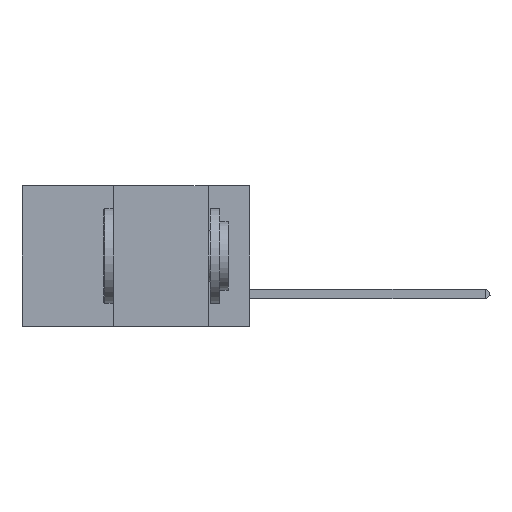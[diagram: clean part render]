
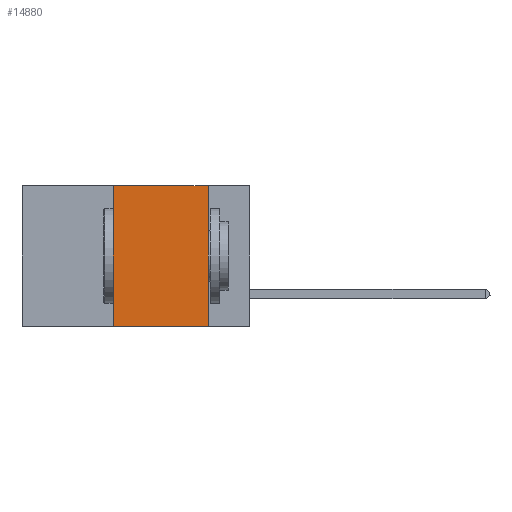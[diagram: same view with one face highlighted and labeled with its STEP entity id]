
A CAD part, left-side view. The second image highlights one B-rep face of the part: STEP entity #14880.
In plain terms, the highlighted planar face has unit normal (-1, 0, 0).
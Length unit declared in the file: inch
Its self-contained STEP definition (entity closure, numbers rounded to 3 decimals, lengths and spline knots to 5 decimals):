
#73 = CARTESIAN_POINT ( 'NONE',  ( 0., 0.11, 0. ) ) ;
#715 = CARTESIAN_POINT ( 'NONE',  ( 0., 0.36, 0. ) ) ;
#4609 = VERTEX_POINT ( 'NONE', #715 ) ;
#6145 = CARTESIAN_POINT ( 'NONE',  ( 0., 0.11, 0. ) ) ;
#11748 = EDGE_CURVE ( 'NONE', #20192, #26360, #21008, .T. ) ;
#11791 = CARTESIAN_POINT ( 'NONE',  ( 0., 0.6, 0. ) ) ;
#12547 = VECTOR ( 'NONE', #41056, 39.37008 ) ;
#13272 = DIRECTION ( 'NONE',  ( 0., -1., 0. ) ) ;
#14880 = ADVANCED_FACE ( 'NONE', ( #40308 ), #36085, .F. ) ;
#18778 = CARTESIAN_POINT ( 'NONE',  ( 0., 0.36, -0.37 ) ) ;
#19255 = CARTESIAN_POINT ( 'NONE',  ( 0., 0.11, -0.37 ) ) ;
#20192 = VERTEX_POINT ( 'NONE', #18778 ) ;
#21008 = LINE ( 'NONE', #24125, #21643 ) ;
#21636 = EDGE_CURVE ( 'NONE', #31765, #26360, #34710, .T. ) ;
#21643 = VECTOR ( 'NONE', #13272, 39.37008 ) ;
#22984 = EDGE_LOOP ( 'NONE', ( #28183, #44640, #44623, #33241 ) ) ;
#24125 = CARTESIAN_POINT ( 'NONE',  ( 0., 0.6, -0.37 ) ) ;
#24415 = AXIS2_PLACEMENT_3D ( 'NONE', #28059, #35913, #43634 ) ;
#26360 = VERTEX_POINT ( 'NONE', #19255 ) ;
#28059 = CARTESIAN_POINT ( 'NONE',  ( 0., 0.6, 0. ) ) ;
#28183 = ORIENTED_EDGE ( 'NONE', *, *, #21636, .F. ) ;
#29440 = CARTESIAN_POINT ( 'NONE',  ( 0., 0.36, 0. ) ) ;
#31687 = VECTOR ( 'NONE', #41578, 39.37008 ) ;
#31765 = VERTEX_POINT ( 'NONE', #73 ) ;
#33241 = ORIENTED_EDGE ( 'NONE', *, *, #11748, .T. ) ;
#34710 = LINE ( 'NONE', #6145, #31687 ) ;
#35913 = DIRECTION ( 'NONE',  ( 1., 0., 0. ) ) ;
#36085 = PLANE ( 'NONE',  #24415 ) ;
#39560 = LINE ( 'NONE', #29440, #12547 ) ;
#39839 = EDGE_CURVE ( 'NONE', #4609, #31765, #43404, .T. ) ;
#40308 = FACE_OUTER_BOUND ( 'NONE', #22984, .T. ) ;
#41056 = DIRECTION ( 'NONE',  ( 0., 0., 1. ) ) ;
#41578 = DIRECTION ( 'NONE',  ( 0., 0., -1. ) ) ;
#43063 = DIRECTION ( 'NONE',  ( 0., -1., 0. ) ) ;
#43404 = LINE ( 'NONE', #11791, #49960 ) ;
#43634 = DIRECTION ( 'NONE',  ( 0., 0., -1. ) ) ;
#44089 = EDGE_CURVE ( 'NONE', #20192, #4609, #39560, .T. ) ;
#44623 = ORIENTED_EDGE ( 'NONE', *, *, #44089, .F. ) ;
#44640 = ORIENTED_EDGE ( 'NONE', *, *, #39839, .F. ) ;
#49960 = VECTOR ( 'NONE', #43063, 39.37008 ) ;
